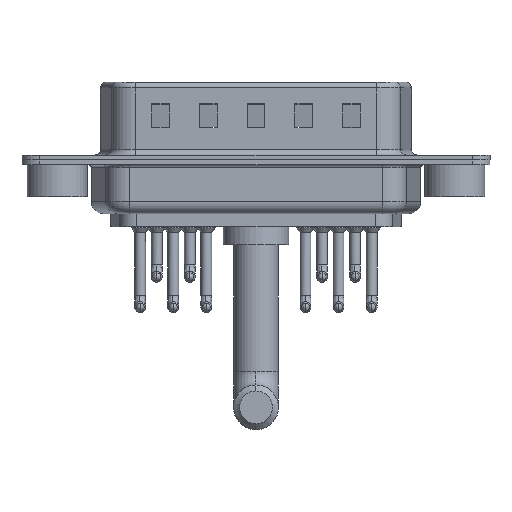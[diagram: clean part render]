
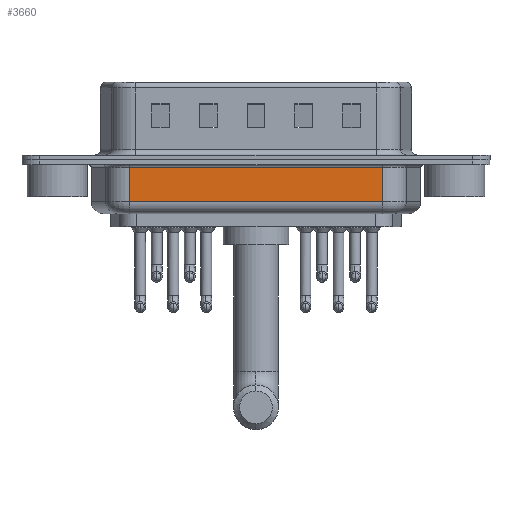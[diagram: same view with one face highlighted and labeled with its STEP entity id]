
A CAD part, front view. The second image highlights one B-rep face of the part: STEP entity #3660.
In plain terms, the highlighted planar face has unit normal (0, -1, 0).
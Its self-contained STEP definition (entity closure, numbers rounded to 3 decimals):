
#642 = DIRECTION ( 'NONE',  ( 0., 1., 0. ) ) ;
#1931 = DIRECTION ( 'NONE',  ( 0., 0., 1. ) ) ;
#2126 = VECTOR ( 'NONE', #1931, 1000. ) ;
#2358 = FACE_OUTER_BOUND ( 'NONE', #4993, .T. ) ;
#2731 = ORIENTED_EDGE ( 'NONE', *, *, #11900, .F. ) ;
#2932 = ORIENTED_EDGE ( 'NONE', *, *, #18553, .T. ) ;
#3573 = CARTESIAN_POINT ( 'NONE',  ( 27.269, -5.35, -3.5 ) ) ;
#3660 = ADVANCED_FACE ( 'NONE', ( #2358 ), #7807, .F. ) ;
#3960 = DIRECTION ( 'NONE',  ( 0., 0., 1. ) ) ;
#4171 = DIRECTION ( 'NONE',  ( 1., 0., 0. ) ) ;
#4993 = EDGE_LOOP ( 'NONE', ( #2731, #16358, #2932, #18168 ) ) ;
#5437 = VERTEX_POINT ( 'NONE', #7240 ) ;
#7240 = CARTESIAN_POINT ( 'NONE',  ( 6.031, -5.35, -0.65 ) ) ;
#7501 = CARTESIAN_POINT ( 'NONE',  ( 6.031, -5.35, -4.5 ) ) ;
#7807 = PLANE ( 'NONE',  #13317 ) ;
#7903 = LINE ( 'NONE', #12780, #14444 ) ;
#8706 = LINE ( 'NONE', #13927, #16023 ) ;
#8903 = CARTESIAN_POINT ( 'NONE',  ( 6.031, -5.35, -3.5 ) ) ;
#10013 = CARTESIAN_POINT ( 'NONE',  ( 27.269, -5.35, -0.65 ) ) ;
#11900 = EDGE_CURVE ( 'NONE', #14489, #5437, #21311, .T. ) ;
#12780 = CARTESIAN_POINT ( 'NONE',  ( 6.031, -5.35, -3.5 ) ) ;
#12796 = CARTESIAN_POINT ( 'NONE',  ( 6.031, -5.35, -4.5 ) ) ;
#13029 = EDGE_CURVE ( 'NONE', #14489, #19327, #7903, .T. ) ;
#13317 = AXIS2_PLACEMENT_3D ( 'NONE', #12796, #642, #3960 ) ;
#13545 = VERTEX_POINT ( 'NONE', #10013 ) ;
#13754 = CARTESIAN_POINT ( 'NONE',  ( 27.269, -5.35, -4.5 ) ) ;
#13927 = CARTESIAN_POINT ( 'NONE',  ( 6.031, -5.35, -0.65 ) ) ;
#14424 = DIRECTION ( 'NONE',  ( 0., 0., 1. ) ) ;
#14444 = VECTOR ( 'NONE', #4171, 1000. ) ;
#14489 = VERTEX_POINT ( 'NONE', #8903 ) ;
#15670 = LINE ( 'NONE', #13754, #2126 ) ;
#16023 = VECTOR ( 'NONE', #20921, 1000. ) ;
#16358 = ORIENTED_EDGE ( 'NONE', *, *, #13029, .T. ) ;
#18168 = ORIENTED_EDGE ( 'NONE', *, *, #21974, .T. ) ;
#18553 = EDGE_CURVE ( 'NONE', #19327, #13545, #15670, .T. ) ;
#19327 = VERTEX_POINT ( 'NONE', #3573 ) ;
#19755 = VECTOR ( 'NONE', #14424, 1000. ) ;
#20921 = DIRECTION ( 'NONE',  ( -1., 0., 0. ) ) ;
#21311 = LINE ( 'NONE', #7501, #19755 ) ;
#21974 = EDGE_CURVE ( 'NONE', #13545, #5437, #8706, .T. ) ;
